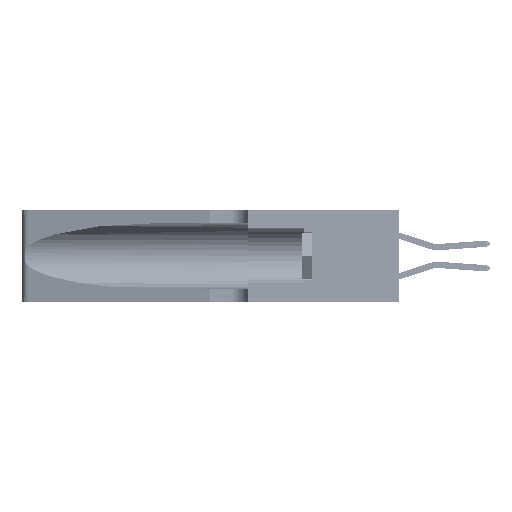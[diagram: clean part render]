
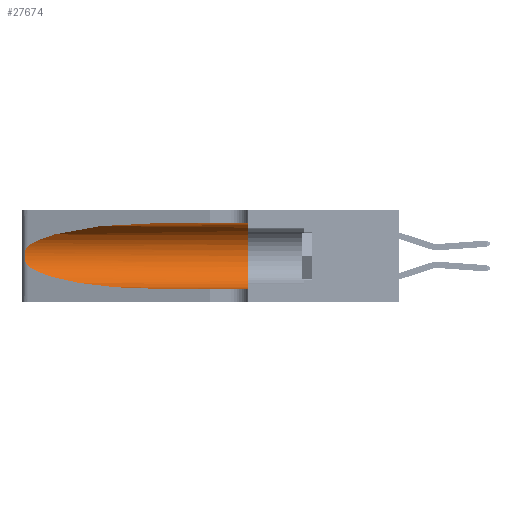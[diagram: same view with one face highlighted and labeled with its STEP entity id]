
A CAD part, left-side view. The second image highlights one B-rep face of the part: STEP entity #27674.
In plain terms, the highlighted cylindrical face has radius 3.308 mm (diameter 6.617 mm), a partial arc.
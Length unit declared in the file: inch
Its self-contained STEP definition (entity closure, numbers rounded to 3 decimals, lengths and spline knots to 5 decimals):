
#318 = CARTESIAN_POINT ( 'NONE',  ( 0.25555, 1.22993, 0.14849 ) ) ;
#533 = FACE_OUTER_BOUND ( 'NONE', #28288, .T. ) ;
#924 = VERTEX_POINT ( 'NONE', #51882 ) ;
#1056 = EDGE_CURVE ( 'NONE', #9282, #47269, #39046, .T. ) ;
#1681 = CARTESIAN_POINT ( 'NONE',  ( 0.2373, 1.15595, 0.28018 ) ) ;
#2014 = EDGE_CURVE ( 'NONE', #47269, #7881, #7597, .T. ) ;
#3692 =( BOUNDED_CURVE ( )  B_SPLINE_CURVE ( 3, ( #22000, #45920, #1681, #30118 ),
 .UNSPECIFIED., .F., .T. ) 
 B_SPLINE_CURVE_WITH_KNOTS ( ( 4, 4 ),
 ( 1.5708, 2.84003 ),
 .UNSPECIFIED. ) 
 CURVE ( )  GEOMETRIC_REPRESENTATION_ITEM ( )  RATIONAL_B_SPLINE_CURVE ( ( 1., 0.87, 0.87, 1. ) ) 
 REPRESENTATION_ITEM ( '' )  );
#4268 = CARTESIAN_POINT ( 'NONE',  ( 0.25487, 1.22718, 0.22369 ) ) ;
#5292 = CARTESIAN_POINT ( 'NONE',  ( 0.25487, 1.22718, 0.14631 ) ) ;
#6365 = DIRECTION ( 'NONE',  ( 0., -1., 0. ) ) ;
#7597 =( BOUNDED_CURVE ( )  B_SPLINE_CURVE ( 3, ( #5292, #33625, #17583, #45598 ),
 .UNSPECIFIED., .F., .F. ) 
 B_SPLINE_CURVE_WITH_KNOTS ( ( 4, 4 ),
 ( 3.44316, 4.71239 ),
 .UNSPECIFIED. ) 
 CURVE ( )  GEOMETRIC_REPRESENTATION_ITEM ( )  RATIONAL_B_SPLINE_CURVE ( ( 1., 0.87, 0.87, 1. ) ) 
 REPRESENTATION_ITEM ( '' )  );
#7881 = VERTEX_POINT ( 'NONE', #13769 ) ;
#8325 = CARTESIAN_POINT ( 'NONE',  ( 0.25787, 1.23484, 0.2124 ) ) ;
#8536 = EDGE_CURVE ( 'NONE', #924, #13515, #22249, .T. ) ;
#9282 = VERTEX_POINT ( 'NONE', #18417 ) ;
#10147 = DIRECTION ( 'NONE',  ( 0., 1., 0. ) ) ;
#11397 = VECTOR ( 'NONE', #41950, 39.37008 ) ;
#12420 = CARTESIAN_POINT ( 'NONE',  ( 0.26018, 1.23835, 0.19895 ) ) ;
#12447 = CIRCLE ( 'NONE', #26369, 0.13025 ) ;
#13215 = VECTOR ( 'NONE', #6365, 39.37008 ) ;
#13515 = VERTEX_POINT ( 'NONE', #20935 ) ;
#13769 = CARTESIAN_POINT ( 'NONE',  ( 0.1305, 0.72297, 0.05475 ) ) ;
#14608 = DIRECTION ( 'NONE',  ( 0., 0., -1. ) ) ;
#16568 = CARTESIAN_POINT ( 'NONE',  ( 0.26075, 1.23896, 0.178 ) ) ;
#16761 = ORIENTED_EDGE ( 'NONE', *, *, #8536, .F. ) ;
#17583 = CARTESIAN_POINT ( 'NONE',  ( 0.18966, 0.96281, 0.05475 ) ) ;
#17954 = CARTESIAN_POINT ( 'NONE',  ( 0.1305, 1.61858, 0.31525 ) ) ;
#18417 = CARTESIAN_POINT ( 'NONE',  ( 0.25487, 1.22718, 0.22369 ) ) ;
#19702 = CARTESIAN_POINT ( 'NONE',  ( 0.25487, 1.22718, 0.14631 ) ) ;
#20667 = CARTESIAN_POINT ( 'NONE',  ( 0.25856, 1.23593, 0.16098 ) ) ;
#20844 = EDGE_CURVE ( 'NONE', #13515, #24267, #12447, .T. ) ;
#20935 = CARTESIAN_POINT ( 'NONE',  ( 0.1305, 0.35, 0.31525 ) ) ;
#20973 = CYLINDRICAL_SURFACE ( 'NONE', #42220, 0.13025 ) ;
#22000 = CARTESIAN_POINT ( 'NONE',  ( 0.1305, 0.72297, 0.31525 ) ) ;
#22147 = EDGE_CURVE ( 'NONE', #924, #9282, #3692, .T. ) ;
#22249 = LINE ( 'NONE', #17954, #11397 ) ;
#24267 = VERTEX_POINT ( 'NONE', #49836 ) ;
#24565 = CARTESIAN_POINT ( 'NONE',  ( 0.25555, 1.22994, 0.2215 ) ) ;
#24743 = CARTESIAN_POINT ( 'NONE',  ( 0.25639, 1.23186, 0.15144 ) ) ;
#26369 = AXIS2_PLACEMENT_3D ( 'NONE', #34368, #10147, #38386 ) ;
#26936 = ORIENTED_EDGE ( 'NONE', *, *, #20844, .F. ) ;
#27674 = ADVANCED_FACE ( 'NONE', ( #533 ), #20973, .F. ) ;
#28288 = EDGE_LOOP ( 'NONE', ( #44384, #36911, #31952, #51807, #26936, #16761 ) ) ;
#28328 = EDGE_CURVE ( 'NONE', #7881, #24267, #33457, .T. ) ;
#28783 = CARTESIAN_POINT ( 'NONE',  ( 0.25487, 1.22718, 0.14631 ) ) ;
#30118 = CARTESIAN_POINT ( 'NONE',  ( 0.25487, 1.22718, 0.22369 ) ) ;
#30672 = CARTESIAN_POINT ( 'NONE',  ( 0.1305, 1.61858, 0.05475 ) ) ;
#31952 = ORIENTED_EDGE ( 'NONE', *, *, #2014, .T. ) ;
#32609 = CARTESIAN_POINT ( 'NONE',  ( 0.25639, 1.23184, 0.21858 ) ) ;
#33457 = LINE ( 'NONE', #30672, #13215 ) ;
#33625 = CARTESIAN_POINT ( 'NONE',  ( 0.2373, 1.15595, 0.08982 ) ) ;
#34368 = CARTESIAN_POINT ( 'NONE',  ( 0.1305, 0.35, 0.185 ) ) ;
#36604 = CARTESIAN_POINT ( 'NONE',  ( 0.25854, 1.2359, 0.20912 ) ) ;
#36911 = ORIENTED_EDGE ( 'NONE', *, *, #1056, .T. ) ;
#38386 = DIRECTION ( 'NONE',  ( 0., 0., 1. ) ) ;
#38903 = DIRECTION ( 'NONE',  ( 0., -1., 0. ) ) ;
#39046 = B_SPLINE_CURVE_WITH_KNOTS ( 'NONE', 3,
 ( #4268, #24565, #32609, #8325, #36604, #12420, #40610, #16568, #44587, #20667, #48595, #24743, #318, #28783 ),
 .UNSPECIFIED., .F., .F.,
 ( 4, 2, 2, 2, 2, 2, 4 ),
 ( 0., 0.00027, 0.00053, 0.00107, 0.0016, 0.00187, 0.00214 ),
 .UNSPECIFIED. ) ;
#40610 = CARTESIAN_POINT ( 'NONE',  ( 0.26075, 1.23896, 0.19203 ) ) ;
#41950 = DIRECTION ( 'NONE',  ( 0., -1., 0. ) ) ;
#42220 = AXIS2_PLACEMENT_3D ( 'NONE', #46707, #38903, #14608 ) ;
#44384 = ORIENTED_EDGE ( 'NONE', *, *, #22147, .T. ) ;
#44587 = CARTESIAN_POINT ( 'NONE',  ( 0.26017, 1.23833, 0.17102 ) ) ;
#45598 = CARTESIAN_POINT ( 'NONE',  ( 0.1305, 0.72297, 0.05475 ) ) ;
#45920 = CARTESIAN_POINT ( 'NONE',  ( 0.18966, 0.96281, 0.31525 ) ) ;
#46707 = CARTESIAN_POINT ( 'NONE',  ( 0.1305, 1.61858, 0.185 ) ) ;
#47269 = VERTEX_POINT ( 'NONE', #19702 ) ;
#48595 = CARTESIAN_POINT ( 'NONE',  ( 0.25789, 1.23486, 0.15765 ) ) ;
#49836 = CARTESIAN_POINT ( 'NONE',  ( 0.1305, 0.35, 0.05475 ) ) ;
#51807 = ORIENTED_EDGE ( 'NONE', *, *, #28328, .T. ) ;
#51882 = CARTESIAN_POINT ( 'NONE',  ( 0.1305, 0.72297, 0.31525 ) ) ;
